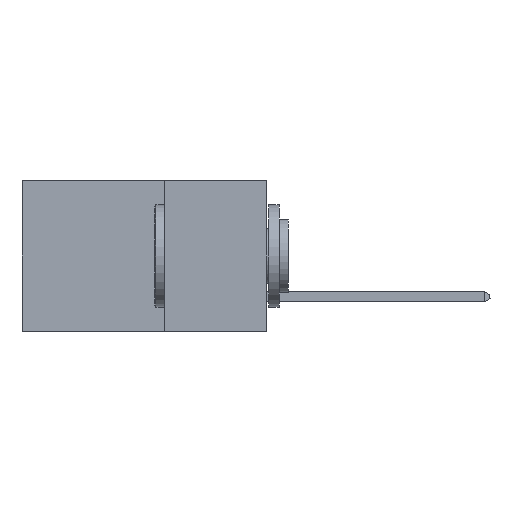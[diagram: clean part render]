
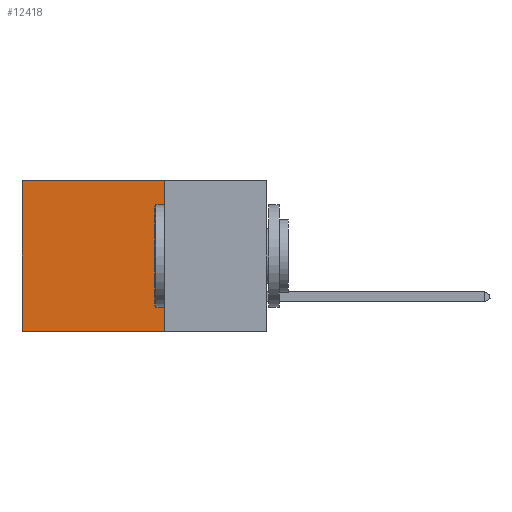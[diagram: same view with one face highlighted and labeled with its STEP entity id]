
A CAD part, left-side view. The second image highlights one B-rep face of the part: STEP entity #12418.
In plain terms, the highlighted planar face has unit normal (-1, 0, 0).
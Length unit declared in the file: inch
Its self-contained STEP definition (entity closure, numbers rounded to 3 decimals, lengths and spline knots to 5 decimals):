
#1138 = ORIENTED_EDGE ( 'NONE', *, *, #12864, .F. ) ;
#1970 = LINE ( 'NONE', #7796, #9487 ) ;
#2677 = PLANE ( 'NONE',  #11773 ) ;
#2900 = CARTESIAN_POINT ( 'NONE',  ( 0.2875, 0.25, 0. ) ) ;
#3291 = VERTEX_POINT ( 'NONE', #11852 ) ;
#5427 = DIRECTION ( 'NONE',  ( 0., 0., -1. ) ) ;
#5647 = CARTESIAN_POINT ( 'NONE',  ( 0.2875, 0.6, -0.37 ) ) ;
#5788 = LINE ( 'NONE', #30743, #30527 ) ;
#6743 = VECTOR ( 'NONE', #7863, 39.37008 ) ;
#7497 = VERTEX_POINT ( 'NONE', #28258 ) ;
#7731 = CARTESIAN_POINT ( 'NONE',  ( 0.2875, 0.25, 0. ) ) ;
#7796 = CARTESIAN_POINT ( 'NONE',  ( 0.2875, 0.25, -0.37 ) ) ;
#7863 = DIRECTION ( 'NONE',  ( 0., 0., -1. ) ) ;
#8467 = EDGE_CURVE ( 'NONE', #3291, #21145, #22114, .T. ) ;
#9487 = VECTOR ( 'NONE', #12527, 39.37008 ) ;
#9651 = ORIENTED_EDGE ( 'NONE', *, *, #8467, .T. ) ;
#9848 = DIRECTION ( 'NONE',  ( 0., 0., -1. ) ) ;
#10331 = VECTOR ( 'NONE', #5427, 39.37008 ) ;
#11773 = AXIS2_PLACEMENT_3D ( 'NONE', #7731, #28873, #9848 ) ;
#11852 = CARTESIAN_POINT ( 'NONE',  ( 0.2875, 0.6, 0. ) ) ;
#12418 = ADVANCED_FACE ( 'NONE', ( #25648 ), #2677, .F. ) ;
#12527 = DIRECTION ( 'NONE',  ( 0., 1., 0. ) ) ;
#12864 = EDGE_CURVE ( 'NONE', #30451, #21145, #1970, .T. ) ;
#13899 = DIRECTION ( 'NONE',  ( 0., 1., 0. ) ) ;
#21145 = VERTEX_POINT ( 'NONE', #5647 ) ;
#22114 = LINE ( 'NONE', #22330, #6743 ) ;
#22330 = CARTESIAN_POINT ( 'NONE',  ( 0.2875, 0.6, 0. ) ) ;
#23076 = EDGE_CURVE ( 'NONE', #7497, #3291, #5788, .T. ) ;
#25648 = FACE_OUTER_BOUND ( 'NONE', #26715, .T. ) ;
#26040 = LINE ( 'NONE', #2900, #10331 ) ;
#26715 = EDGE_LOOP ( 'NONE', ( #9651, #1138, #27352, #27633 ) ) ;
#27350 = EDGE_CURVE ( 'NONE', #7497, #30451, #26040, .T. ) ;
#27352 = ORIENTED_EDGE ( 'NONE', *, *, #27350, .F. ) ;
#27402 = CARTESIAN_POINT ( 'NONE',  ( 0.2875, 0.25, -0.37 ) ) ;
#27633 = ORIENTED_EDGE ( 'NONE', *, *, #23076, .T. ) ;
#28258 = CARTESIAN_POINT ( 'NONE',  ( 0.2875, 0.25, 0. ) ) ;
#28873 = DIRECTION ( 'NONE',  ( 1., 0., 0. ) ) ;
#30451 = VERTEX_POINT ( 'NONE', #27402 ) ;
#30527 = VECTOR ( 'NONE', #13899, 39.37008 ) ;
#30743 = CARTESIAN_POINT ( 'NONE',  ( 0.2875, 0.25, 0. ) ) ;
